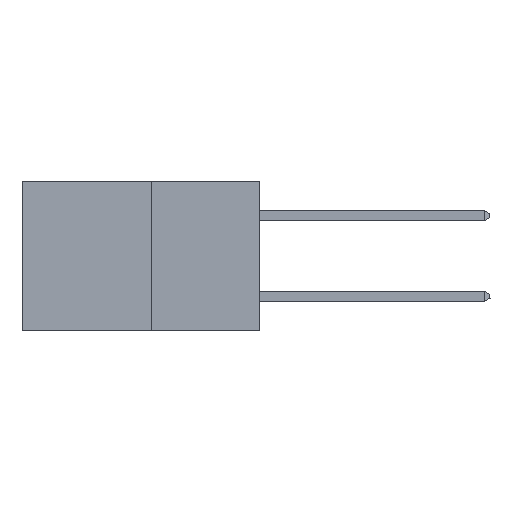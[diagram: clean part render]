
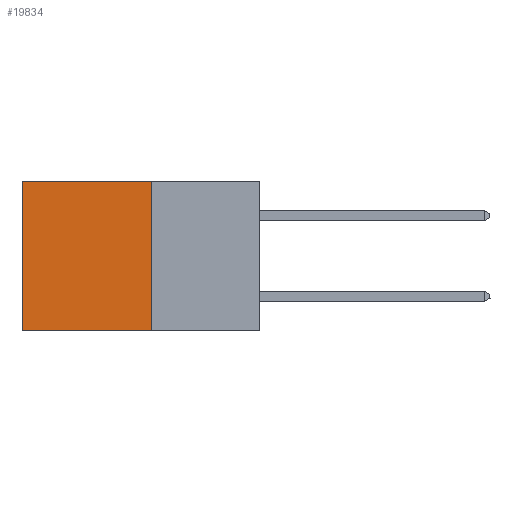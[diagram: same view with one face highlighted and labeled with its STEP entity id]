
A CAD part, left-side view. The second image highlights one B-rep face of the part: STEP entity #19834.
In plain terms, the highlighted planar face has unit normal (-1, 0, 0).
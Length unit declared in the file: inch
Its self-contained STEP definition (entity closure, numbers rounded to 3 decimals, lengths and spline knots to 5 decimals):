
#2627 = DIRECTION ( 'NONE',  ( 0., 0., -1. ) ) ;
#3216 = VERTEX_POINT ( 'NONE', #8579 ) ;
#5361 = VECTOR ( 'NONE', #6286, 39.37008 ) ;
#5878 = LINE ( 'NONE', #26169, #23213 ) ;
#6286 = DIRECTION ( 'NONE',  ( 0., 1., 0. ) ) ;
#6484 = VERTEX_POINT ( 'NONE', #20328 ) ;
#7373 = EDGE_CURVE ( 'NONE', #3216, #18324, #26276, .T. ) ;
#7770 = VECTOR ( 'NONE', #14706, 39.37008 ) ;
#8579 = CARTESIAN_POINT ( 'NONE',  ( 0.277, 0.27, 0. ) ) ;
#8652 = ORIENTED_EDGE ( 'NONE', *, *, #9676, .F. ) ;
#8836 = CARTESIAN_POINT ( 'NONE',  ( 0.277, 0.27, -0.37 ) ) ;
#9676 = EDGE_CURVE ( 'NONE', #12012, #6484, #5878, .T. ) ;
#10128 = CARTESIAN_POINT ( 'NONE',  ( 0.277, 0.27, -0.37 ) ) ;
#10613 = CARTESIAN_POINT ( 'NONE',  ( 0.277, 0.27, -0.37 ) ) ;
#11544 = DIRECTION ( 'NONE',  ( 0., 1., 0. ) ) ;
#12012 = VERTEX_POINT ( 'NONE', #10613 ) ;
#12558 = CARTESIAN_POINT ( 'NONE',  ( 0.277, 0.59, -0.37 ) ) ;
#12679 = LINE ( 'NONE', #12558, #7770 ) ;
#13075 = PLANE ( 'NONE',  #16599 ) ;
#14670 = ORIENTED_EDGE ( 'NONE', *, *, #19689, .F. ) ;
#14706 = DIRECTION ( 'NONE',  ( 0., 0., -1. ) ) ;
#15193 = DIRECTION ( 'NONE',  ( 1., 0., 0. ) ) ;
#16599 = AXIS2_PLACEMENT_3D ( 'NONE', #8836, #15193, #2627 ) ;
#17817 = ORIENTED_EDGE ( 'NONE', *, *, #7373, .T. ) ;
#18323 = ORIENTED_EDGE ( 'NONE', *, *, #24327, .T. ) ;
#18324 = VERTEX_POINT ( 'NONE', #23425 ) ;
#19689 = EDGE_CURVE ( 'NONE', #3216, #12012, #26062, .T. ) ;
#19834 = ADVANCED_FACE ( 'NONE', ( #22806 ), #13075, .F. ) ;
#20328 = CARTESIAN_POINT ( 'NONE',  ( 0.277, 0.59, -0.37 ) ) ;
#20676 = DIRECTION ( 'NONE',  ( 0., 0., -1. ) ) ;
#20918 = CARTESIAN_POINT ( 'NONE',  ( 0.277, 0.27, 0. ) ) ;
#22315 = EDGE_LOOP ( 'NONE', ( #18323, #8652, #14670, #17817 ) ) ;
#22806 = FACE_OUTER_BOUND ( 'NONE', #22315, .T. ) ;
#23213 = VECTOR ( 'NONE', #11544, 39.37008 ) ;
#23425 = CARTESIAN_POINT ( 'NONE',  ( 0.277, 0.59, 0. ) ) ;
#24327 = EDGE_CURVE ( 'NONE', #18324, #6484, #12679, .T. ) ;
#25405 = VECTOR ( 'NONE', #20676, 39.37008 ) ;
#26062 = LINE ( 'NONE', #10128, #25405 ) ;
#26169 = CARTESIAN_POINT ( 'NONE',  ( 0.277, 0.27, -0.37 ) ) ;
#26276 = LINE ( 'NONE', #20918, #5361 ) ;
